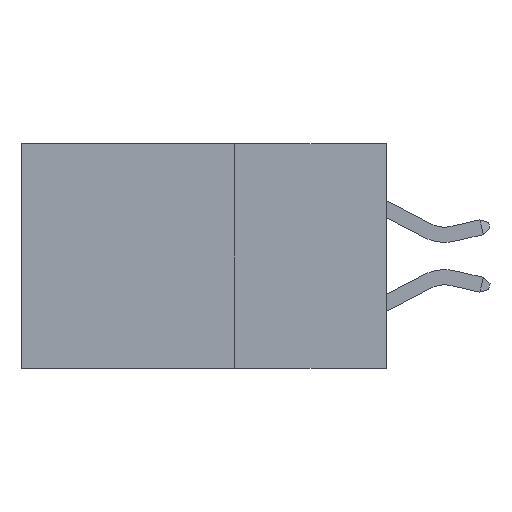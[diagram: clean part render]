
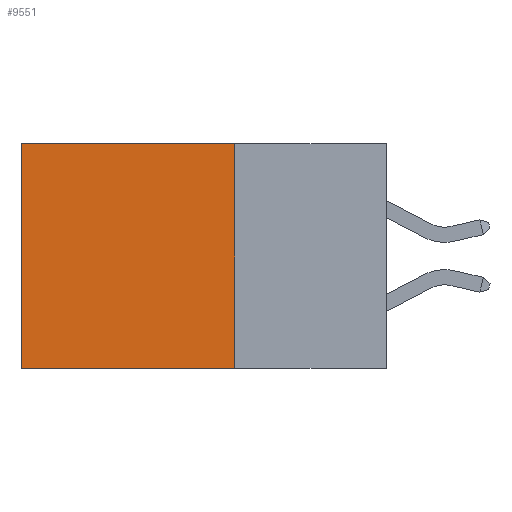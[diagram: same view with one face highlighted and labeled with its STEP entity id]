
A CAD part, left-side view. The second image highlights one B-rep face of the part: STEP entity #9551.
In plain terms, the highlighted planar face has unit normal (-1, 0, 0).
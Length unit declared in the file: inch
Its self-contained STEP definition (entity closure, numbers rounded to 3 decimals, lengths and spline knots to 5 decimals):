
#119 = DIRECTION ( 'NONE',  ( 0., 0., -1. ) ) ;
#233 = ORIENTED_EDGE ( 'NONE', *, *, #518, .F. ) ;
#488 = CARTESIAN_POINT ( 'NONE',  ( 0.2615, 0.25, -0.37 ) ) ;
#518 = EDGE_CURVE ( 'NONE', #6342, #3480, #9063, .T. ) ;
#1026 = CARTESIAN_POINT ( 'NONE',  ( 0.2615, 0.25, -0.37 ) ) ;
#1209 = CARTESIAN_POINT ( 'NONE',  ( 0.2615, 0.25, 0. ) ) ;
#1516 = VECTOR ( 'NONE', #2116, 39.37008 ) ;
#2027 = EDGE_CURVE ( 'NONE', #8326, #6342, #4769, .T. ) ;
#2116 = DIRECTION ( 'NONE',  ( 0., 0., -1. ) ) ;
#2118 = CARTESIAN_POINT ( 'NONE',  ( 0.2615, 0.25, -0.37 ) ) ;
#2134 = VECTOR ( 'NONE', #4958, 39.37008 ) ;
#2236 = VECTOR ( 'NONE', #10848, 39.37008 ) ;
#2613 = EDGE_LOOP ( 'NONE', ( #7181, #233, #4609, #3408 ) ) ;
#3189 = PLANE ( 'NONE',  #9333 ) ;
#3314 = EDGE_CURVE ( 'NONE', #8326, #3779, #4092, .T. ) ;
#3408 = ORIENTED_EDGE ( 'NONE', *, *, #3314, .T. ) ;
#3480 = VERTEX_POINT ( 'NONE', #8380 ) ;
#3779 = VERTEX_POINT ( 'NONE', #5703 ) ;
#4092 = LINE ( 'NONE', #9724, #8196 ) ;
#4609 = ORIENTED_EDGE ( 'NONE', *, *, #2027, .F. ) ;
#4769 = LINE ( 'NONE', #488, #2236 ) ;
#4958 = DIRECTION ( 'NONE',  ( 0., 1., 0. ) ) ;
#5231 = LINE ( 'NONE', #9879, #1516 ) ;
#5703 = CARTESIAN_POINT ( 'NONE',  ( 0.2615, 0.6, 0. ) ) ;
#5803 = DIRECTION ( 'NONE',  ( 1., 0., 0. ) ) ;
#6342 = VERTEX_POINT ( 'NONE', #1026 ) ;
#7181 = ORIENTED_EDGE ( 'NONE', *, *, #7348, .T. ) ;
#7348 = EDGE_CURVE ( 'NONE', #3779, #3480, #5231, .T. ) ;
#8190 = CARTESIAN_POINT ( 'NONE',  ( 0.2615, 0.25, -0.37 ) ) ;
#8196 = VECTOR ( 'NONE', #10226, 39.37008 ) ;
#8326 = VERTEX_POINT ( 'NONE', #1209 ) ;
#8380 = CARTESIAN_POINT ( 'NONE',  ( 0.2615, 0.6, -0.37 ) ) ;
#8496 = FACE_OUTER_BOUND ( 'NONE', #2613, .T. ) ;
#9063 = LINE ( 'NONE', #8190, #2134 ) ;
#9333 = AXIS2_PLACEMENT_3D ( 'NONE', #2118, #5803, #119 ) ;
#9551 = ADVANCED_FACE ( 'NONE', ( #8496 ), #3189, .F. ) ;
#9724 = CARTESIAN_POINT ( 'NONE',  ( 0.2615, 0.25, 0. ) ) ;
#9879 = CARTESIAN_POINT ( 'NONE',  ( 0.2615, 0.6, -0.37 ) ) ;
#10226 = DIRECTION ( 'NONE',  ( 0., 1., 0. ) ) ;
#10848 = DIRECTION ( 'NONE',  ( 0., 0., -1. ) ) ;
